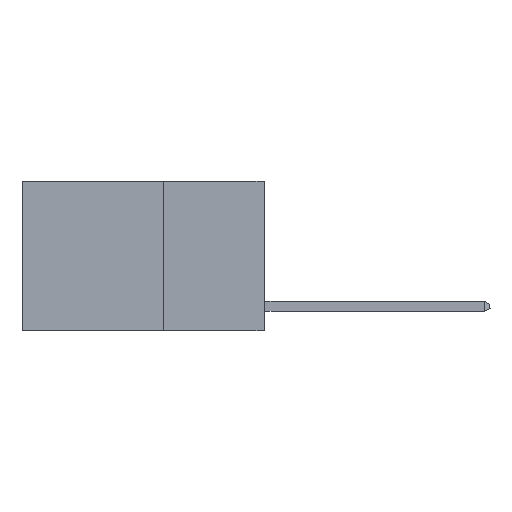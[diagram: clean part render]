
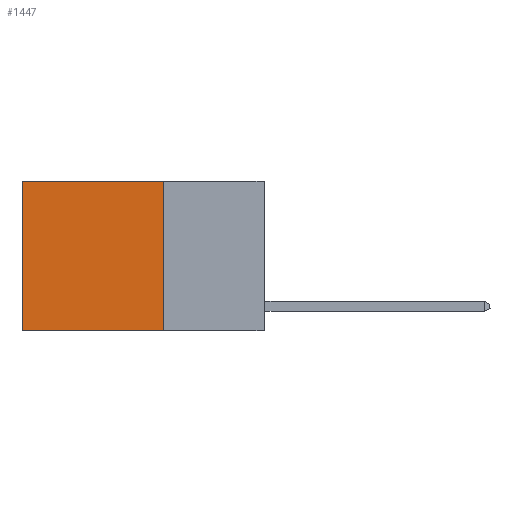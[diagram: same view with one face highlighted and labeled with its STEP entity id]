
A CAD part, left-side view. The second image highlights one B-rep face of the part: STEP entity #1447.
In plain terms, the highlighted planar face has unit normal (-1, 0, 0).
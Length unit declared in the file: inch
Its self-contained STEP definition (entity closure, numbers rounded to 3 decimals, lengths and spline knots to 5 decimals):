
#25 = DIRECTION ( 'NONE',  ( 0., 1., 0. ) ) ;
#127 = EDGE_LOOP ( 'NONE', ( #9992, #580, #2047, #2052 ) ) ;
#176 = VERTEX_POINT ( 'NONE', #517 ) ;
#410 = CARTESIAN_POINT ( 'NONE',  ( 0.2625, 0.25, 0. ) ) ;
#517 = CARTESIAN_POINT ( 'NONE',  ( 0.2625, 0.6, 0. ) ) ;
#580 = ORIENTED_EDGE ( 'NONE', *, *, #4041, .F. ) ;
#927 = CARTESIAN_POINT ( 'NONE',  ( 0.2625, 0.25, -0.37 ) ) ;
#1447 = ADVANCED_FACE ( 'NONE', ( #2029 ), #8388, .F. ) ;
#1705 = CARTESIAN_POINT ( 'NONE',  ( 0.2625, 0.25, 0. ) ) ;
#1739 = CARTESIAN_POINT ( 'NONE',  ( 0.2625, 0.25, 0. ) ) ;
#1823 = LINE ( 'NONE', #927, #4671 ) ;
#2029 = FACE_OUTER_BOUND ( 'NONE', #127, .T. ) ;
#2047 = ORIENTED_EDGE ( 'NONE', *, *, #5929, .F. ) ;
#2052 = ORIENTED_EDGE ( 'NONE', *, *, #2995, .T. ) ;
#2995 = EDGE_CURVE ( 'NONE', #3933, #176, #4539, .T. ) ;
#3453 = DIRECTION ( 'NONE',  ( 0., 0., -1. ) ) ;
#3933 = VERTEX_POINT ( 'NONE', #1705 ) ;
#4041 = EDGE_CURVE ( 'NONE', #7135, #7646, #1823, .T. ) ;
#4356 = LINE ( 'NONE', #6240, #5300 ) ;
#4539 = LINE ( 'NONE', #1739, #11630 ) ;
#4666 = DIRECTION ( 'NONE',  ( 0., 0., -1. ) ) ;
#4671 = VECTOR ( 'NONE', #25, 39.37008 ) ;
#5300 = VECTOR ( 'NONE', #3453, 39.37008 ) ;
#5656 = CARTESIAN_POINT ( 'NONE',  ( 0.2625, 0.25, 0. ) ) ;
#5765 = CARTESIAN_POINT ( 'NONE',  ( 0.2625, 0.25, -0.37 ) ) ;
#5929 = EDGE_CURVE ( 'NONE', #3933, #7135, #7641, .T. ) ;
#6191 = DIRECTION ( 'NONE',  ( 0., 1., 0. ) ) ;
#6240 = CARTESIAN_POINT ( 'NONE',  ( 0.2625, 0.6, 0. ) ) ;
#6747 = CARTESIAN_POINT ( 'NONE',  ( 0.2625, 0.6, -0.37 ) ) ;
#6761 = DIRECTION ( 'NONE',  ( 0., 0., -1. ) ) ;
#6950 = AXIS2_PLACEMENT_3D ( 'NONE', #5656, #10027, #4666 ) ;
#7135 = VERTEX_POINT ( 'NONE', #5765 ) ;
#7641 = LINE ( 'NONE', #410, #8842 ) ;
#7646 = VERTEX_POINT ( 'NONE', #6747 ) ;
#8388 = PLANE ( 'NONE',  #6950 ) ;
#8842 = VECTOR ( 'NONE', #6761, 39.37008 ) ;
#9506 = EDGE_CURVE ( 'NONE', #176, #7646, #4356, .T. ) ;
#9992 = ORIENTED_EDGE ( 'NONE', *, *, #9506, .T. ) ;
#10027 = DIRECTION ( 'NONE',  ( 1., 0., 0. ) ) ;
#11630 = VECTOR ( 'NONE', #6191, 39.37008 ) ;
